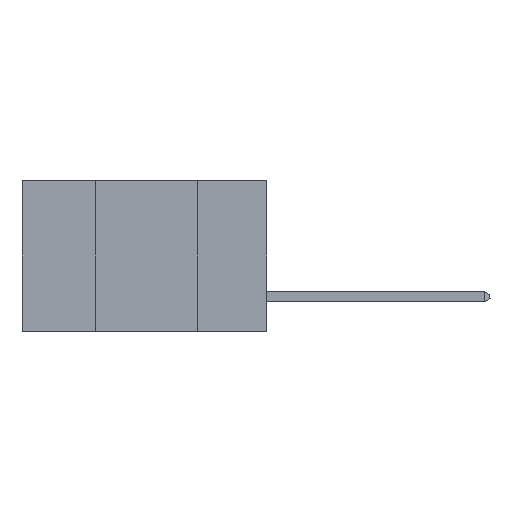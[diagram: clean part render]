
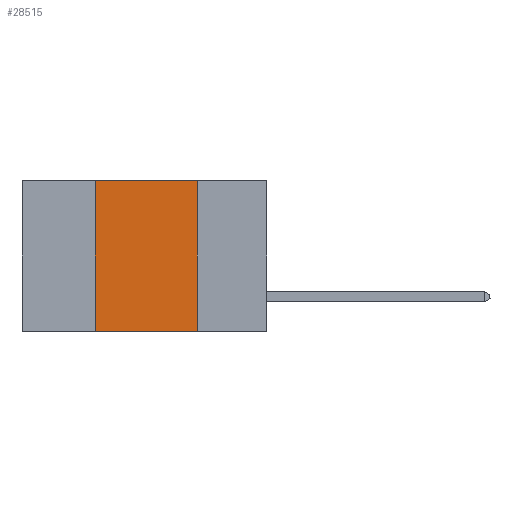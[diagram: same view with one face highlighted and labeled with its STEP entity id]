
A CAD part, left-side view. The second image highlights one B-rep face of the part: STEP entity #28515.
In plain terms, the highlighted planar face has unit normal (-1, 0, 0).
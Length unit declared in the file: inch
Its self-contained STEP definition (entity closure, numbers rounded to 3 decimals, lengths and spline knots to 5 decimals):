
#26 = CARTESIAN_POINT ( 'NONE',  ( 0., 0.6, 0. ) ) ;
#719 = CARTESIAN_POINT ( 'NONE',  ( 0., 0.17, 0. ) ) ;
#1946 = ORIENTED_EDGE ( 'NONE', *, *, #32684, .F. ) ;
#2123 = DIRECTION ( 'NONE',  ( 0., 0., 1. ) ) ;
#2736 = VERTEX_POINT ( 'NONE', #719 ) ;
#3243 = EDGE_CURVE ( 'NONE', #26138, #2736, #9139, .T. ) ;
#3528 = DIRECTION ( 'NONE',  ( 0., 0., -1. ) ) ;
#3992 = CARTESIAN_POINT ( 'NONE',  ( 0., 0.17, 0. ) ) ;
#5127 = ORIENTED_EDGE ( 'NONE', *, *, #3243, .F. ) ;
#7093 = ORIENTED_EDGE ( 'NONE', *, *, #23206, .T. ) ;
#7818 = ORIENTED_EDGE ( 'NONE', *, *, #24272, .F. ) ;
#9139 = LINE ( 'NONE', #28164, #17630 ) ;
#10334 = LINE ( 'NONE', #30734, #27759 ) ;
#11127 = LINE ( 'NONE', #3992, #28525 ) ;
#15925 = EDGE_LOOP ( 'NONE', ( #7818, #5127, #1946, #7093 ) ) ;
#16626 = CARTESIAN_POINT ( 'NONE',  ( 0., 0.6, -0.37 ) ) ;
#17630 = VECTOR ( 'NONE', #30871, 39.37008 ) ;
#18096 = VECTOR ( 'NONE', #32271, 39.37008 ) ;
#18116 = DIRECTION ( 'NONE',  ( 1., 0., 0. ) ) ;
#18320 = VERTEX_POINT ( 'NONE', #26647 ) ;
#21147 = DIRECTION ( 'NONE',  ( 0., 0., -1. ) ) ;
#21724 = FACE_OUTER_BOUND ( 'NONE', #15925, .T. ) ;
#23206 = EDGE_CURVE ( 'NONE', #29054, #18320, #24968, .T. ) ;
#24272 = EDGE_CURVE ( 'NONE', #2736, #18320, #11127, .T. ) ;
#24968 = LINE ( 'NONE', #16626, #18096 ) ;
#25772 = PLANE ( 'NONE',  #25831 ) ;
#25831 = AXIS2_PLACEMENT_3D ( 'NONE', #26, #18116, #21147 ) ;
#26138 = VERTEX_POINT ( 'NONE', #31084 ) ;
#26647 = CARTESIAN_POINT ( 'NONE',  ( 0., 0.17, -0.37 ) ) ;
#27759 = VECTOR ( 'NONE', #2123, 39.37008 ) ;
#28164 = CARTESIAN_POINT ( 'NONE',  ( 0., 0.6, 0. ) ) ;
#28515 = ADVANCED_FACE ( 'NONE', ( #21724 ), #25772, .F. ) ;
#28525 = VECTOR ( 'NONE', #3528, 39.37008 ) ;
#29054 = VERTEX_POINT ( 'NONE', #32893 ) ;
#30734 = CARTESIAN_POINT ( 'NONE',  ( 0., 0.42, 0. ) ) ;
#30871 = DIRECTION ( 'NONE',  ( 0., -1., 0. ) ) ;
#31084 = CARTESIAN_POINT ( 'NONE',  ( 0., 0.42, 0. ) ) ;
#32271 = DIRECTION ( 'NONE',  ( 0., -1., 0. ) ) ;
#32684 = EDGE_CURVE ( 'NONE', #29054, #26138, #10334, .T. ) ;
#32893 = CARTESIAN_POINT ( 'NONE',  ( 0., 0.42, -0.37 ) ) ;
